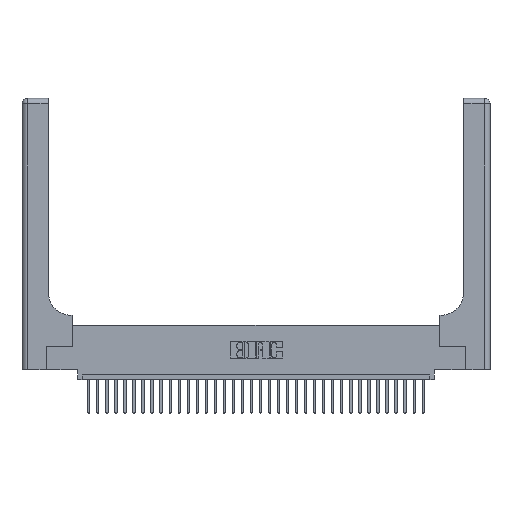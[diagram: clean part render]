
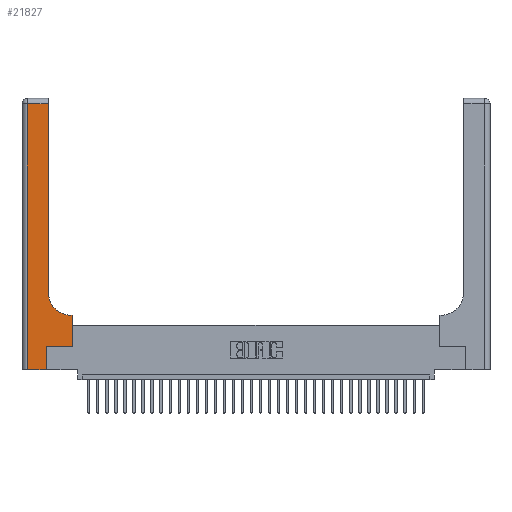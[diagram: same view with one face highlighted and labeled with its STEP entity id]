
A CAD part, top view. The second image highlights one B-rep face of the part: STEP entity #21827.
In plain terms, the highlighted planar face has unit normal (0, 0, 1).
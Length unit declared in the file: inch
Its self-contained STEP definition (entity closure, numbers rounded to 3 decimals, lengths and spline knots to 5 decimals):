
#176 = CARTESIAN_POINT ( 'NONE',  ( 0., 0., 0.37 ) ) ;
#413 = LINE ( 'NONE', #14264, #3345 ) ;
#460 = VERTEX_POINT ( 'NONE', #10269 ) ;
#532 = DIRECTION ( 'NONE',  ( 0., 1., 0. ) ) ;
#618 = VERTEX_POINT ( 'NONE', #8115 ) ;
#2175 = VERTEX_POINT ( 'NONE', #14491 ) ;
#2805 = CARTESIAN_POINT ( 'NONE',  ( 0.5415, 0.6, 0.37 ) ) ;
#3345 = VECTOR ( 'NONE', #22082, 39.37008 ) ;
#4675 = EDGE_CURVE ( 'NONE', #12522, #10915, #33783, .T. ) ;
#6201 = ORIENTED_EDGE ( 'NONE', *, *, #28834, .T. ) ;
#6653 = EDGE_CURVE ( 'NONE', #29739, #2175, #27676, .T. ) ;
#7458 = FACE_OUTER_BOUND ( 'NONE', #27438, .T. ) ;
#7511 = VERTEX_POINT ( 'NONE', #22081 ) ;
#7760 = AXIS2_PLACEMENT_3D ( 'NONE', #32220, #11176, #24393 ) ;
#8115 = CARTESIAN_POINT ( 'NONE',  ( 0.06, 0., 0.37 ) ) ;
#8125 = DIRECTION ( 'NONE',  ( -1., 0., 0. ) ) ;
#8143 = CARTESIAN_POINT ( 'NONE',  ( 0.269, 0.25, 0.37 ) ) ;
#8172 = DIRECTION ( 'NONE',  ( 0., 1., 0. ) ) ;
#8188 = ORIENTED_EDGE ( 'NONE', *, *, #6653, .T. ) ;
#8440 = ORIENTED_EDGE ( 'NONE', *, *, #15712, .T. ) ;
#8853 = VECTOR ( 'NONE', #32292, 39.37008 ) ;
#9625 = ORIENTED_EDGE ( 'NONE', *, *, #27220, .T. ) ;
#9726 = CARTESIAN_POINT ( 'NONE',  ( 0.269, 0.25, 0.37 ) ) ;
#9866 = ORIENTED_EDGE ( 'NONE', *, *, #14095, .T. ) ;
#10236 = LINE ( 'NONE', #176, #30988 ) ;
#10269 = CARTESIAN_POINT ( 'NONE',  ( 0.5585, 0.25, 0.37 ) ) ;
#10500 = DIRECTION ( 'NONE',  ( 1., 0., 0. ) ) ;
#10798 = CARTESIAN_POINT ( 'NONE',  ( 0.269, 0., 0.37 ) ) ;
#10915 = VERTEX_POINT ( 'NONE', #2805 ) ;
#11176 = DIRECTION ( 'NONE',  ( 0., 0., -1. ) ) ;
#11198 = CARTESIAN_POINT ( 'NONE',  ( 0.06, 3., 0.37 ) ) ;
#11429 = LINE ( 'NONE', #11198, #18504 ) ;
#11575 = VERTEX_POINT ( 'NONE', #9726 ) ;
#11602 = EDGE_CURVE ( 'NONE', #16986, #11575, #17971, .T. ) ;
#12039 = CARTESIAN_POINT ( 'NONE',  ( 0.2915, 0.85, 0.37 ) ) ;
#12396 = ORIENTED_EDGE ( 'NONE', *, *, #4675, .T. ) ;
#12522 = VERTEX_POINT ( 'NONE', #22922 ) ;
#13449 = VECTOR ( 'NONE', #8172, 39.37008 ) ;
#13458 = VECTOR ( 'NONE', #8125, 39.37008 ) ;
#14095 = EDGE_CURVE ( 'NONE', #7511, #618, #11429, .T. ) ;
#14134 = DIRECTION ( 'NONE',  ( -1., 0., 0. ) ) ;
#14264 = CARTESIAN_POINT ( 'NONE',  ( 0., 2.94, 0.37 ) ) ;
#14491 = CARTESIAN_POINT ( 'NONE',  ( 0.2915, 2.94, 0.37 ) ) ;
#14574 = EDGE_CURVE ( 'NONE', #10915, #29739, #23443, .T. ) ;
#14586 = EDGE_CURVE ( 'NONE', #460, #12522, #26373, .T. ) ;
#15324 = ORIENTED_EDGE ( 'NONE', *, *, #14574, .T. ) ;
#15712 = EDGE_CURVE ( 'NONE', #2175, #7511, #413, .T. ) ;
#15914 = CARTESIAN_POINT ( 'NONE',  ( 0.269, 0., 0.37 ) ) ;
#16042 = CARTESIAN_POINT ( 'NONE',  ( 0.2915, 3., 0.37 ) ) ;
#16480 = CARTESIAN_POINT ( 'NONE',  ( 0.2915, 0.6, 0.37 ) ) ;
#16517 = DIRECTION ( 'NONE',  ( 0., 0., -1. ) ) ;
#16524 = DIRECTION ( 'NONE',  ( 0., -1., 0. ) ) ;
#16986 = VERTEX_POINT ( 'NONE', #10798 ) ;
#17971 = LINE ( 'NONE', #15914, #13449 ) ;
#18504 = VECTOR ( 'NONE', #16524, 39.37008 ) ;
#18629 = VECTOR ( 'NONE', #18720, 39.37008 ) ;
#18720 = DIRECTION ( 'NONE',  ( 1., 0., 0. ) ) ;
#19056 = CARTESIAN_POINT ( 'NONE',  ( 0.5585, 0.25, 0.37 ) ) ;
#19188 = PLANE ( 'NONE',  #20142 ) ;
#19453 = LINE ( 'NONE', #8143, #18629 ) ;
#20142 = AXIS2_PLACEMENT_3D ( 'NONE', #32450, #16517, #14134 ) ;
#21827 = ADVANCED_FACE ( 'NONE', ( #7458 ), #19188, .F. ) ;
#22081 = CARTESIAN_POINT ( 'NONE',  ( 0.06, 2.94, 0.37 ) ) ;
#22082 = DIRECTION ( 'NONE',  ( -1., 0., 0. ) ) ;
#22922 = CARTESIAN_POINT ( 'NONE',  ( 0.5585, 0.6, 0.37 ) ) ;
#23443 = CIRCLE ( 'NONE', #7760, 0.25 ) ;
#24393 = DIRECTION ( 'NONE',  ( 1., 0., 0. ) ) ;
#26373 = LINE ( 'NONE', #19056, #28424 ) ;
#27220 = EDGE_CURVE ( 'NONE', #11575, #460, #19453, .T. ) ;
#27438 = EDGE_LOOP ( 'NONE', ( #8188, #8440, #9866, #6201, #30344, #9625, #34392, #12396, #15324 ) ) ;
#27676 = LINE ( 'NONE', #16042, #8853 ) ;
#28424 = VECTOR ( 'NONE', #532, 39.37008 ) ;
#28834 = EDGE_CURVE ( 'NONE', #618, #16986, #10236, .T. ) ;
#29739 = VERTEX_POINT ( 'NONE', #12039 ) ;
#30344 = ORIENTED_EDGE ( 'NONE', *, *, #11602, .T. ) ;
#30988 = VECTOR ( 'NONE', #10500, 39.37008 ) ;
#32220 = CARTESIAN_POINT ( 'NONE',  ( 0.5415, 0.85, 0.37 ) ) ;
#32292 = DIRECTION ( 'NONE',  ( 0., 1., 0. ) ) ;
#32450 = CARTESIAN_POINT ( 'NONE',  ( 0., 3., 0.37 ) ) ;
#33783 = LINE ( 'NONE', #16480, #13458 ) ;
#34392 = ORIENTED_EDGE ( 'NONE', *, *, #14586, .T. ) ;
